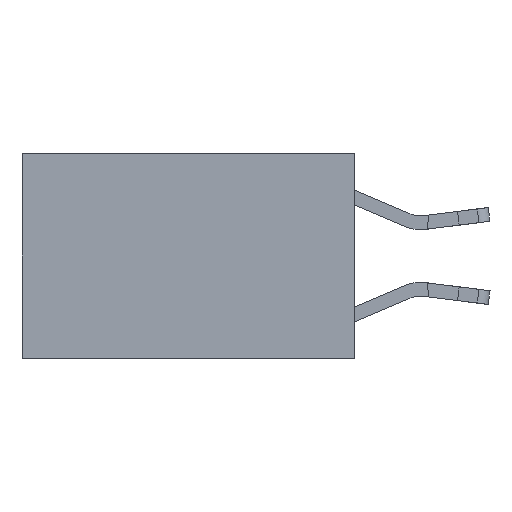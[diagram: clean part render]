
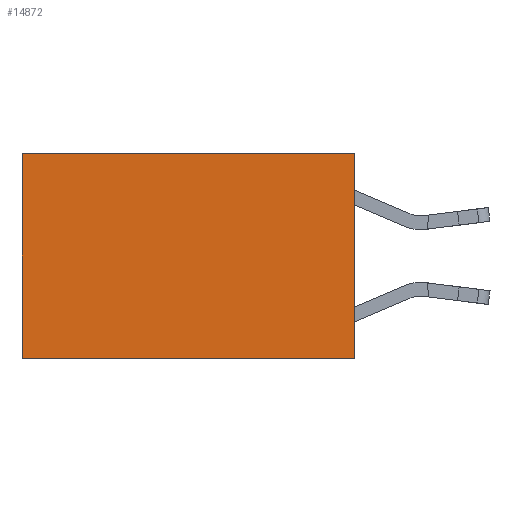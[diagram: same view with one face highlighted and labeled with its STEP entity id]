
A CAD part, left-side view. The second image highlights one B-rep face of the part: STEP entity #14872.
In plain terms, the highlighted planar face has unit normal (-1, 0, 0).
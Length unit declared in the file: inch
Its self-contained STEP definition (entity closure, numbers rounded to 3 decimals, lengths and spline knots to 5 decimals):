
#1621 = CARTESIAN_POINT ( 'NONE',  ( 0.2625, 0., 0. ) ) ;
#2207 = VERTEX_POINT ( 'NONE', #22943 ) ;
#2517 = CARTESIAN_POINT ( 'NONE',  ( 0.2625, 0., 0. ) ) ;
#3280 = ORIENTED_EDGE ( 'NONE', *, *, #3511, .T. ) ;
#3511 = EDGE_CURVE ( 'NONE', #2207, #13785, #5438, .T. ) ;
#3666 = VERTEX_POINT ( 'NONE', #15826 ) ;
#3949 = DIRECTION ( 'NONE',  ( 0., 0., -1. ) ) ;
#4524 = ORIENTED_EDGE ( 'NONE', *, *, #20581, .F. ) ;
#5438 = LINE ( 'NONE', #11546, #15552 ) ;
#5704 = DIRECTION ( 'NONE',  ( 0., 0., -1. ) ) ;
#6811 = EDGE_CURVE ( 'NONE', #13387, #2207, #19767, .T. ) ;
#7248 = AXIS2_PLACEMENT_3D ( 'NONE', #17248, #20953, #9718 ) ;
#7329 = FACE_OUTER_BOUND ( 'NONE', #14885, .T. ) ;
#7801 = PLANE ( 'NONE',  #7248 ) ;
#8530 = CARTESIAN_POINT ( 'NONE',  ( 0.2625, 0.6, -0.37 ) ) ;
#9718 = DIRECTION ( 'NONE',  ( 0., 0., -1. ) ) ;
#11546 = CARTESIAN_POINT ( 'NONE',  ( 0.2625, 0.6, 0. ) ) ;
#11804 = VECTOR ( 'NONE', #5704, 39.37008 ) ;
#12055 = CARTESIAN_POINT ( 'NONE',  ( 0.2625, 0., -0.37 ) ) ;
#13010 = EDGE_CURVE ( 'NONE', #3666, #13785, #20674, .T. ) ;
#13387 = VERTEX_POINT ( 'NONE', #1621 ) ;
#13785 = VERTEX_POINT ( 'NONE', #8530 ) ;
#14212 = VECTOR ( 'NONE', #19547, 39.37008 ) ;
#14872 = ADVANCED_FACE ( 'NONE', ( #7329 ), #7801, .F. ) ;
#14885 = EDGE_LOOP ( 'NONE', ( #3280, #20032, #4524, #17941 ) ) ;
#15552 = VECTOR ( 'NONE', #3949, 39.37008 ) ;
#15740 = VECTOR ( 'NONE', #19502, 39.37008 ) ;
#15826 = CARTESIAN_POINT ( 'NONE',  ( 0.2625, 0., -0.37 ) ) ;
#17006 = CARTESIAN_POINT ( 'NONE',  ( 0.2625, 0., 0. ) ) ;
#17248 = CARTESIAN_POINT ( 'NONE',  ( 0.2625, 0., 0. ) ) ;
#17941 = ORIENTED_EDGE ( 'NONE', *, *, #6811, .T. ) ;
#19502 = DIRECTION ( 'NONE',  ( 0., 1., 0. ) ) ;
#19547 = DIRECTION ( 'NONE',  ( 0., 1., 0. ) ) ;
#19767 = LINE ( 'NONE', #2517, #14212 ) ;
#20032 = ORIENTED_EDGE ( 'NONE', *, *, #13010, .F. ) ;
#20581 = EDGE_CURVE ( 'NONE', #13387, #3666, #21719, .T. ) ;
#20674 = LINE ( 'NONE', #12055, #15740 ) ;
#20953 = DIRECTION ( 'NONE',  ( 1., 0., 0. ) ) ;
#21719 = LINE ( 'NONE', #17006, #11804 ) ;
#22943 = CARTESIAN_POINT ( 'NONE',  ( 0.2625, 0.6, 0. ) ) ;
